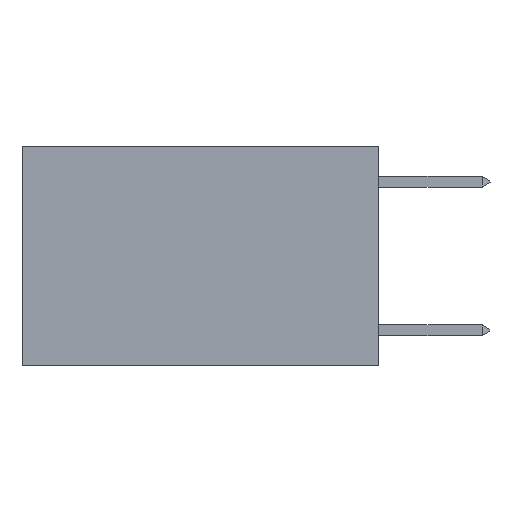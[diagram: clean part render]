
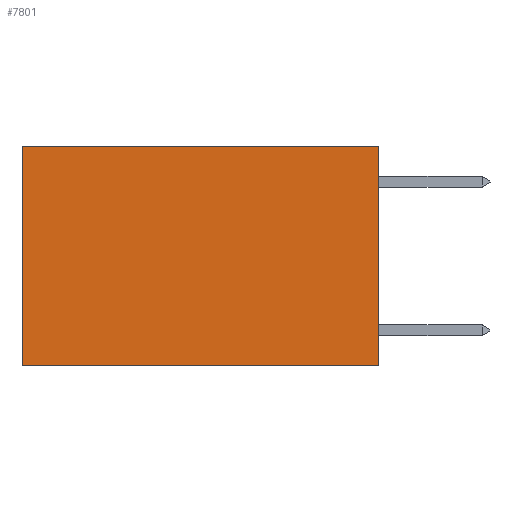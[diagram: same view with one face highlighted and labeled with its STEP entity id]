
A CAD part, left-side view. The second image highlights one B-rep face of the part: STEP entity #7801.
In plain terms, the highlighted planar face has unit normal (-1, 0, 0).
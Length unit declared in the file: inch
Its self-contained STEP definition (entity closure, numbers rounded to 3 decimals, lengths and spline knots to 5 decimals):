
#99 = CARTESIAN_POINT ( 'NONE',  ( 0.2625, 0.6, 0. ) ) ;
#275 = ORIENTED_EDGE ( 'NONE', *, *, #5598, .F. ) ;
#322 = ORIENTED_EDGE ( 'NONE', *, *, #6780, .T. ) ;
#975 = CARTESIAN_POINT ( 'NONE',  ( 0.2625, 0.6, 0. ) ) ;
#1855 = CARTESIAN_POINT ( 'NONE',  ( 0.2625, 0., 0. ) ) ;
#1927 = EDGE_LOOP ( 'NONE', ( #322, #275, #2510, #2909 ) ) ;
#2415 = DIRECTION ( 'NONE',  ( 0., 0., -1. ) ) ;
#2510 = ORIENTED_EDGE ( 'NONE', *, *, #8395, .F. ) ;
#2909 = ORIENTED_EDGE ( 'NONE', *, *, #6525, .T. ) ;
#3063 = LINE ( 'NONE', #8313, #7136 ) ;
#3622 = CARTESIAN_POINT ( 'NONE',  ( 0.2625, 0., -0.37 ) ) ;
#3905 = VERTEX_POINT ( 'NONE', #1855 ) ;
#4261 = DIRECTION ( 'NONE',  ( 0., 0., -1. ) ) ;
#4316 = VECTOR ( 'NONE', #5522, 39.37008 ) ;
#4327 = LINE ( 'NONE', #3622, #8952 ) ;
#4547 = LINE ( 'NONE', #6880, #6033 ) ;
#5177 = DIRECTION ( 'NONE',  ( 1., 0., 0. ) ) ;
#5522 = DIRECTION ( 'NONE',  ( 0., 0., -1. ) ) ;
#5598 = EDGE_CURVE ( 'NONE', #8808, #6505, #4327, .T. ) ;
#5895 = AXIS2_PLACEMENT_3D ( 'NONE', #6598, #5177, #4261 ) ;
#6033 = VECTOR ( 'NONE', #8235, 39.37008 ) ;
#6265 = LINE ( 'NONE', #975, #4316 ) ;
#6505 = VERTEX_POINT ( 'NONE', #9479 ) ;
#6525 = EDGE_CURVE ( 'NONE', #3905, #9231, #4547, .T. ) ;
#6598 = CARTESIAN_POINT ( 'NONE',  ( 0.2625, 0., 0. ) ) ;
#6699 = FACE_OUTER_BOUND ( 'NONE', #1927, .T. ) ;
#6780 = EDGE_CURVE ( 'NONE', #9231, #6505, #6265, .T. ) ;
#6880 = CARTESIAN_POINT ( 'NONE',  ( 0.2625, 0., 0. ) ) ;
#7136 = VECTOR ( 'NONE', #2415, 39.37008 ) ;
#7293 = DIRECTION ( 'NONE',  ( 0., 1., 0. ) ) ;
#7519 = CARTESIAN_POINT ( 'NONE',  ( 0.2625, 0., -0.37 ) ) ;
#7801 = ADVANCED_FACE ( 'NONE', ( #6699 ), #8875, .F. ) ;
#8235 = DIRECTION ( 'NONE',  ( 0., 1., 0. ) ) ;
#8313 = CARTESIAN_POINT ( 'NONE',  ( 0.2625, 0., 0. ) ) ;
#8395 = EDGE_CURVE ( 'NONE', #3905, #8808, #3063, .T. ) ;
#8808 = VERTEX_POINT ( 'NONE', #7519 ) ;
#8875 = PLANE ( 'NONE',  #5895 ) ;
#8952 = VECTOR ( 'NONE', #7293, 39.37008 ) ;
#9231 = VERTEX_POINT ( 'NONE', #99 ) ;
#9479 = CARTESIAN_POINT ( 'NONE',  ( 0.2625, 0.6, -0.37 ) ) ;
